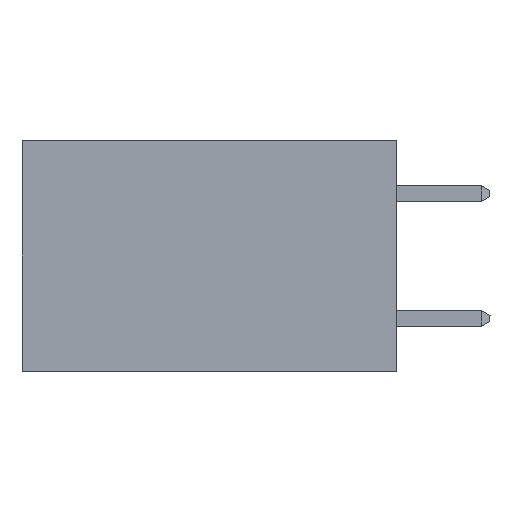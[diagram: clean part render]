
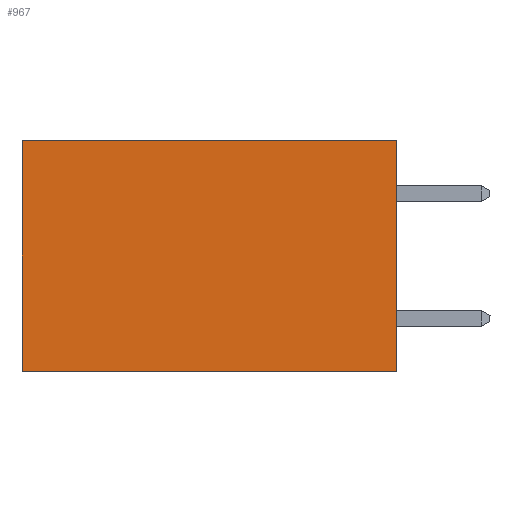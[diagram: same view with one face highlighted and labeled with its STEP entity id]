
A CAD part, left-side view. The second image highlights one B-rep face of the part: STEP entity #967.
In plain terms, the highlighted planar face has unit normal (-1, 0, 0).
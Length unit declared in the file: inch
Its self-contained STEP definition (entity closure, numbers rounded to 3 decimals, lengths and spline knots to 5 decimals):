
#114 = EDGE_CURVE ( 'NONE', #10355, #5180, #5087, .T. ) ;
#622 = ORIENTED_EDGE ( 'NONE', *, *, #2038, .T. ) ;
#670 = DIRECTION ( 'NONE',  ( 0., 0., -1. ) ) ;
#967 = ADVANCED_FACE ( 'NONE', ( #6311 ), #1166, .F. ) ;
#1166 = PLANE ( 'NONE',  #2741 ) ;
#1233 = ORIENTED_EDGE ( 'NONE', *, *, #9775, .F. ) ;
#1263 = EDGE_CURVE ( 'NONE', #3063, #7997, #10093, .T. ) ;
#2038 = EDGE_CURVE ( 'NONE', #7997, #5180, #4192, .T. ) ;
#2612 = VECTOR ( 'NONE', #8591, 39.37008 ) ;
#2741 = AXIS2_PLACEMENT_3D ( 'NONE', #6870, #10122, #8409 ) ;
#2848 = ORIENTED_EDGE ( 'NONE', *, *, #1263, .T. ) ;
#3063 = VERTEX_POINT ( 'NONE', #6927 ) ;
#3363 = LINE ( 'NONE', #4535, #2612 ) ;
#3923 = DIRECTION ( 'NONE',  ( 0., 1., 0. ) ) ;
#4192 = LINE ( 'NONE', #4681, #9818 ) ;
#4535 = CARTESIAN_POINT ( 'NONE',  ( 0.298, 0., 0. ) ) ;
#4681 = CARTESIAN_POINT ( 'NONE',  ( 0.298, 0.6, 0. ) ) ;
#4813 = CARTESIAN_POINT ( 'NONE',  ( 0.298, 0., -0.37 ) ) ;
#4835 = CARTESIAN_POINT ( 'NONE',  ( 0.298, 0., -0.37 ) ) ;
#4876 = CARTESIAN_POINT ( 'NONE',  ( 0.298, 0.6, 0. ) ) ;
#4966 = CARTESIAN_POINT ( 'NONE',  ( 0.298, 0., 0. ) ) ;
#5036 = ORIENTED_EDGE ( 'NONE', *, *, #114, .F. ) ;
#5087 = LINE ( 'NONE', #4813, #8824 ) ;
#5180 = VERTEX_POINT ( 'NONE', #7515 ) ;
#6311 = FACE_OUTER_BOUND ( 'NONE', #6617, .T. ) ;
#6617 = EDGE_LOOP ( 'NONE', ( #622, #5036, #1233, #2848 ) ) ;
#6870 = CARTESIAN_POINT ( 'NONE',  ( 0.298, 0., 0. ) ) ;
#6927 = CARTESIAN_POINT ( 'NONE',  ( 0.298, 0., 0. ) ) ;
#7443 = VECTOR ( 'NONE', #3923, 39.37008 ) ;
#7515 = CARTESIAN_POINT ( 'NONE',  ( 0.298, 0.6, -0.37 ) ) ;
#7997 = VERTEX_POINT ( 'NONE', #4876 ) ;
#8108 = DIRECTION ( 'NONE',  ( 0., 1., 0. ) ) ;
#8409 = DIRECTION ( 'NONE',  ( 0., 0., -1. ) ) ;
#8591 = DIRECTION ( 'NONE',  ( 0., 0., -1. ) ) ;
#8824 = VECTOR ( 'NONE', #8108, 39.37008 ) ;
#9775 = EDGE_CURVE ( 'NONE', #3063, #10355, #3363, .T. ) ;
#9818 = VECTOR ( 'NONE', #670, 39.37008 ) ;
#10093 = LINE ( 'NONE', #4966, #7443 ) ;
#10122 = DIRECTION ( 'NONE',  ( 1., 0., 0. ) ) ;
#10355 = VERTEX_POINT ( 'NONE', #4835 ) ;
